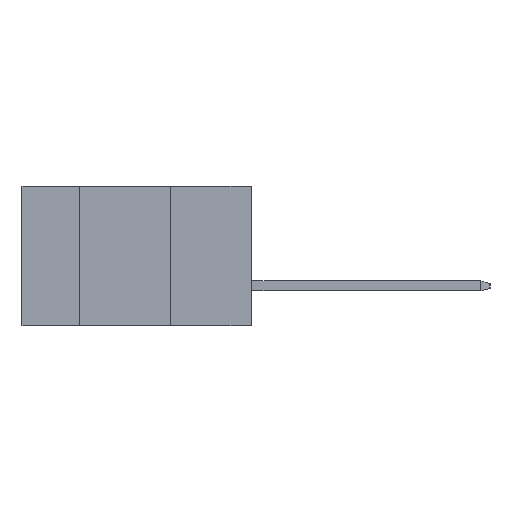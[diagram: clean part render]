
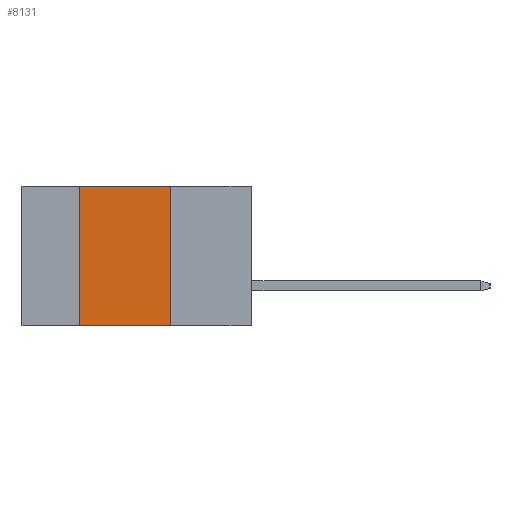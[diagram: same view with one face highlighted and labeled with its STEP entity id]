
A CAD part, left-side view. The second image highlights one B-rep face of the part: STEP entity #8131.
In plain terms, the highlighted planar face has unit normal (-1, 0, 0).
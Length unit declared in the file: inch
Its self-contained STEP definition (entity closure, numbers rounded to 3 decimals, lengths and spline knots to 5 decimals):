
#360 = VECTOR ( 'NONE', #822, 39.37008 ) ;
#640 = EDGE_CURVE ( 'NONE', #6627, #8598, #1111, .T. ) ;
#726 = ORIENTED_EDGE ( 'NONE', *, *, #2035, .T. ) ;
#822 = DIRECTION ( 'NONE',  ( 0., -1., 0. ) ) ;
#1111 = LINE ( 'NONE', #8532, #6130 ) ;
#1484 = VERTEX_POINT ( 'NONE', #4964 ) ;
#1608 = LINE ( 'NONE', #7477, #360 ) ;
#1814 = CARTESIAN_POINT ( 'NONE',  ( 0., 0.54, -0.437 ) ) ;
#1963 = EDGE_CURVE ( 'NONE', #8561, #1484, #2765, .T. ) ;
#2035 = EDGE_CURVE ( 'NONE', #6627, #1484, #4272, .T. ) ;
#2094 = DIRECTION ( 'NONE',  ( 0., 0., -1. ) ) ;
#2765 = LINE ( 'NONE', #7320, #7435 ) ;
#2809 = CARTESIAN_POINT ( 'NONE',  ( 0., 0.72, -0.437 ) ) ;
#2822 = PLANE ( 'NONE',  #4213 ) ;
#3016 = CARTESIAN_POINT ( 'NONE',  ( 0., 0.254, 0. ) ) ;
#4078 = DIRECTION ( 'NONE',  ( 0., 0., 1. ) ) ;
#4213 = AXIS2_PLACEMENT_3D ( 'NONE', #5793, #8780, #2094 ) ;
#4272 = LINE ( 'NONE', #2809, #7279 ) ;
#4955 = DIRECTION ( 'NONE',  ( 0., 0., -1. ) ) ;
#4964 = CARTESIAN_POINT ( 'NONE',  ( 0., 0.254, -0.437 ) ) ;
#5652 = ORIENTED_EDGE ( 'NONE', *, *, #1963, .F. ) ;
#5793 = CARTESIAN_POINT ( 'NONE',  ( 0., 0.72, 0. ) ) ;
#5989 = CARTESIAN_POINT ( 'NONE',  ( 0., 0.54, 0. ) ) ;
#6130 = VECTOR ( 'NONE', #4078, 39.37008 ) ;
#6599 = EDGE_CURVE ( 'NONE', #8598, #8561, #1608, .T. ) ;
#6627 = VERTEX_POINT ( 'NONE', #1814 ) ;
#7264 = DIRECTION ( 'NONE',  ( 0., -1., 0. ) ) ;
#7279 = VECTOR ( 'NONE', #7264, 39.37008 ) ;
#7320 = CARTESIAN_POINT ( 'NONE',  ( 0., 0.254, -0.437 ) ) ;
#7435 = VECTOR ( 'NONE', #4955, 39.37008 ) ;
#7477 = CARTESIAN_POINT ( 'NONE',  ( 0., 0.72, 0. ) ) ;
#7673 = ORIENTED_EDGE ( 'NONE', *, *, #6599, .F. ) ;
#8131 = ADVANCED_FACE ( 'NONE', ( #9451 ), #2822, .F. ) ;
#8532 = CARTESIAN_POINT ( 'NONE',  ( 0., 0.54, -0.437 ) ) ;
#8561 = VERTEX_POINT ( 'NONE', #3016 ) ;
#8598 = VERTEX_POINT ( 'NONE', #5989 ) ;
#8780 = DIRECTION ( 'NONE',  ( 1., 0., 0. ) ) ;
#8991 = ORIENTED_EDGE ( 'NONE', *, *, #640, .F. ) ;
#9451 = FACE_OUTER_BOUND ( 'NONE', #9456, .T. ) ;
#9456 = EDGE_LOOP ( 'NONE', ( #5652, #7673, #8991, #726 ) ) ;
